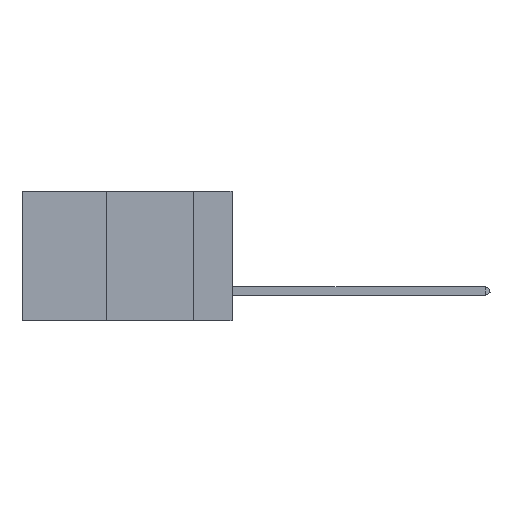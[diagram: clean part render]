
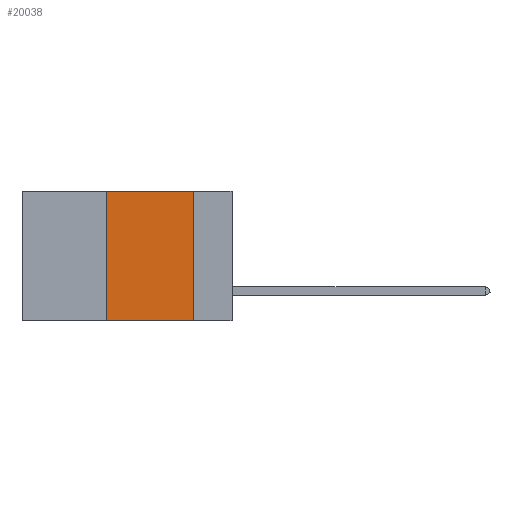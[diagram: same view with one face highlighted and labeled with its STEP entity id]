
A CAD part, left-side view. The second image highlights one B-rep face of the part: STEP entity #20038.
In plain terms, the highlighted planar face has unit normal (-1, 0, 0).
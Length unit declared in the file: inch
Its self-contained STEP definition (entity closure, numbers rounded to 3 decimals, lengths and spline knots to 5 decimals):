
#166 = LINE ( 'NONE', #16670, #22868 ) ;
#1947 = VECTOR ( 'NONE', #25603, 39.37008 ) ;
#3600 = CARTESIAN_POINT ( 'NONE',  ( 0., 0.36, 0. ) ) ;
#3921 = ORIENTED_EDGE ( 'NONE', *, *, #24581, .F. ) ;
#4029 = FACE_OUTER_BOUND ( 'NONE', #6654, .T. ) ;
#5792 = DIRECTION ( 'NONE',  ( 0., 0., 1. ) ) ;
#6654 = EDGE_LOOP ( 'NONE', ( #3921, #15751, #7118, #11846 ) ) ;
#6657 = VERTEX_POINT ( 'NONE', #17712 ) ;
#7050 = LINE ( 'NONE', #14769, #10681 ) ;
#7118 = ORIENTED_EDGE ( 'NONE', *, *, #14539, .F. ) ;
#7949 = VERTEX_POINT ( 'NONE', #22317 ) ;
#10681 = VECTOR ( 'NONE', #14853, 39.37008 ) ;
#11369 = PLANE ( 'NONE',  #19369 ) ;
#11846 = ORIENTED_EDGE ( 'NONE', *, *, #25184, .T. ) ;
#12042 = CARTESIAN_POINT ( 'NONE',  ( 0., 0.36, -0.37 ) ) ;
#13509 = CARTESIAN_POINT ( 'NONE',  ( 0., 0.6, 0. ) ) ;
#13831 = VERTEX_POINT ( 'NONE', #12042 ) ;
#14539 = EDGE_CURVE ( 'NONE', #13831, #6657, #18115, .T. ) ;
#14769 = CARTESIAN_POINT ( 'NONE',  ( 0., 0.6, -0.37 ) ) ;
#14853 = DIRECTION ( 'NONE',  ( 0., -1., 0. ) ) ;
#15119 = LINE ( 'NONE', #21383, #1947 ) ;
#15751 = ORIENTED_EDGE ( 'NONE', *, *, #16017, .F. ) ;
#16017 = EDGE_CURVE ( 'NONE', #6657, #18175, #15119, .T. ) ;
#16670 = CARTESIAN_POINT ( 'NONE',  ( 0., 0.11, 0. ) ) ;
#17518 = DIRECTION ( 'NONE',  ( 0., 0., -1. ) ) ;
#17712 = CARTESIAN_POINT ( 'NONE',  ( 0., 0.36, 0. ) ) ;
#18115 = LINE ( 'NONE', #3600, #18784 ) ;
#18175 = VERTEX_POINT ( 'NONE', #26175 ) ;
#18784 = VECTOR ( 'NONE', #5792, 39.37008 ) ;
#19369 = AXIS2_PLACEMENT_3D ( 'NONE', #13509, #23578, #17518 ) ;
#20038 = ADVANCED_FACE ( 'NONE', ( #4029 ), #11369, .F. ) ;
#21383 = CARTESIAN_POINT ( 'NONE',  ( 0., 0.6, 0. ) ) ;
#22317 = CARTESIAN_POINT ( 'NONE',  ( 0., 0.11, -0.37 ) ) ;
#22868 = VECTOR ( 'NONE', #25186, 39.37008 ) ;
#23578 = DIRECTION ( 'NONE',  ( 1., 0., 0. ) ) ;
#24581 = EDGE_CURVE ( 'NONE', #18175, #7949, #166, .T. ) ;
#25184 = EDGE_CURVE ( 'NONE', #13831, #7949, #7050, .T. ) ;
#25186 = DIRECTION ( 'NONE',  ( 0., 0., -1. ) ) ;
#25603 = DIRECTION ( 'NONE',  ( 0., -1., 0. ) ) ;
#26175 = CARTESIAN_POINT ( 'NONE',  ( 0., 0.11, 0. ) ) ;
